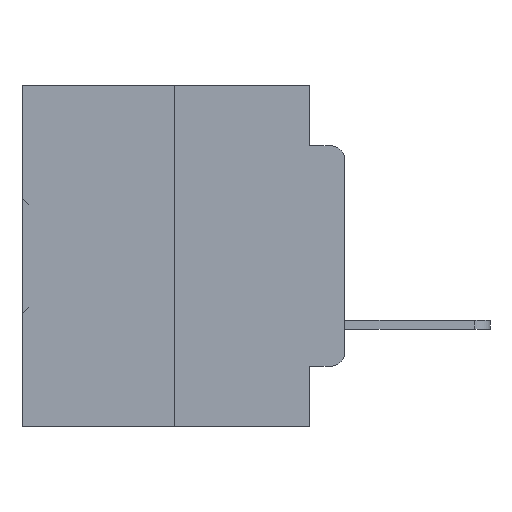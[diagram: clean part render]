
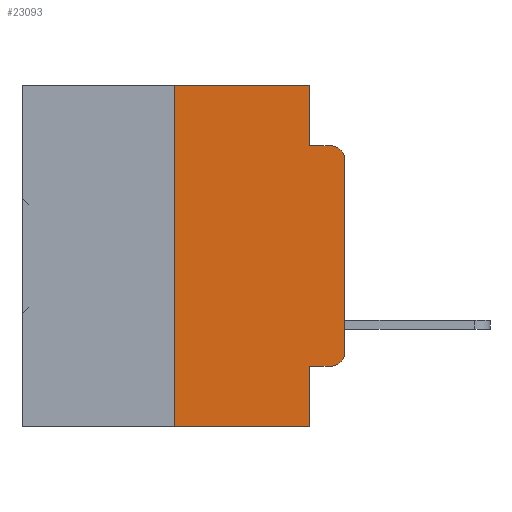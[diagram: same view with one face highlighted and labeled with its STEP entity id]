
A CAD part, left-side view. The second image highlights one B-rep face of the part: STEP entity #23093.
In plain terms, the highlighted planar face has unit normal (-1, 0, 0).
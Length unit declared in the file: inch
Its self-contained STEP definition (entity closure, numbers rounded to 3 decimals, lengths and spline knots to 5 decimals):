
#101 = ORIENTED_EDGE ( 'NONE', *, *, #20485, .T. ) ;
#163 = EDGE_CURVE ( 'NONE', #13387, #16653, #19277, .T. ) ;
#534 = ORIENTED_EDGE ( 'NONE', *, *, #12224, .T. ) ;
#1407 = ORIENTED_EDGE ( 'NONE', *, *, #3550, .F. ) ;
#1460 = LINE ( 'NONE', #19119, #8581 ) ;
#1593 = CARTESIAN_POINT ( 'NONE',  ( 0., 0.051, -0.5 ) ) ;
#1614 = ORIENTED_EDGE ( 'NONE', *, *, #21613, .F. ) ;
#1692 = ORIENTED_EDGE ( 'NONE', *, *, #24259, .F. ) ;
#1952 = ORIENTED_EDGE ( 'NONE', *, *, #17841, .F. ) ;
#2042 = ORIENTED_EDGE ( 'NONE', *, *, #13165, .T. ) ;
#2542 = DIRECTION ( 'NONE',  ( 0., 0., -1. ) ) ;
#2817 = ORIENTED_EDGE ( 'NONE', *, *, #163, .F. ) ;
#2893 = ORIENTED_EDGE ( 'NONE', *, *, #14076, .T. ) ;
#3377 = ORIENTED_EDGE ( 'NONE', *, *, #25380, .T. ) ;
#3550 = EDGE_CURVE ( 'NONE', #28048, #8764, #31536, .T. ) ;
#4096 = CARTESIAN_POINT ( 'NONE',  ( 0., 0.051, -0.0885 ) ) ;
#4329 = VECTOR ( 'NONE', #29502, 39.37008 ) ;
#5026 = CARTESIAN_POINT ( 'NONE',  ( 0., 0.02, -0.4115 ) ) ;
#5465 = CARTESIAN_POINT ( 'NONE',  ( 0., 0.051, -0.0885 ) ) ;
#6001 = VECTOR ( 'NONE', #16373, 39.37008 ) ;
#6758 = CARTESIAN_POINT ( 'NONE',  ( 0., 0.25, -0.5 ) ) ;
#6966 = CARTESIAN_POINT ( 'NONE',  ( 0., 0.051, 0. ) ) ;
#7599 = FACE_OUTER_BOUND ( 'NONE', #13425, .T. ) ;
#8366 = CARTESIAN_POINT ( 'NONE',  ( 0., 0.051, 0. ) ) ;
#8581 = VECTOR ( 'NONE', #27427, 39.37008 ) ;
#8764 = VERTEX_POINT ( 'NONE', #12356 ) ;
#8953 = VECTOR ( 'NONE', #23841, 39.37008 ) ;
#9687 = CARTESIAN_POINT ( 'NONE',  ( 0., 0., -0.3915 ) ) ;
#9900 = LINE ( 'NONE', #29376, #8953 ) ;
#11595 = CARTESIAN_POINT ( 'NONE',  ( 0., 0.02, -0.3915 ) ) ;
#11869 = VERTEX_POINT ( 'NONE', #6758 ) ;
#12214 = CARTESIAN_POINT ( 'NONE',  ( 0., 0.473, 0. ) ) ;
#12224 = EDGE_CURVE ( 'NONE', #22399, #8764, #19757, .T. ) ;
#12356 = CARTESIAN_POINT ( 'NONE',  ( 0., 0.02, -0.0885 ) ) ;
#12906 = CARTESIAN_POINT ( 'NONE',  ( 0., 0.473, 0. ) ) ;
#13165 = EDGE_CURVE ( 'NONE', #11869, #16653, #34197, .T. ) ;
#13387 = VERTEX_POINT ( 'NONE', #35613 ) ;
#13425 = EDGE_LOOP ( 'NONE', ( #101, #534, #1407, #1614, #1692, #1952, #2042, #2817, #2893, #3377 ) ) ;
#13742 = LINE ( 'NONE', #32911, #6001 ) ;
#14076 = EDGE_CURVE ( 'NONE', #13387, #35954, #20490, .T. ) ;
#14393 = DIRECTION ( 'NONE',  ( 0., 0., -1. ) ) ;
#14446 = CARTESIAN_POINT ( 'NONE',  ( 0., 0.051, -0.4115 ) ) ;
#15016 = DIRECTION ( 'NONE',  ( 0., -1., 0. ) ) ;
#15813 = DIRECTION ( 'NONE',  ( 0., 0., -1. ) ) ;
#16373 = DIRECTION ( 'NONE',  ( 0., 0., 1. ) ) ;
#16653 = VERTEX_POINT ( 'NONE', #1593 ) ;
#17252 = DIRECTION ( 'NONE',  ( 0., -1., 0. ) ) ;
#17841 = EDGE_CURVE ( 'NONE', #11869, #24341, #13742, .T. ) ;
#19119 = CARTESIAN_POINT ( 'NONE',  ( 0., 0., 0. ) ) ;
#19135 = VERTEX_POINT ( 'NONE', #6966 ) ;
#19277 = LINE ( 'NONE', #8366, #25858 ) ;
#19757 = CIRCLE ( 'NONE', #25357, 0.02 ) ;
#19957 = DIRECTION ( 'NONE',  ( -1., 0., 0. ) ) ;
#20037 = VECTOR ( 'NONE', #15016, 39.37008 ) ;
#20485 = EDGE_CURVE ( 'NONE', #29592, #22399, #1460, .T. ) ;
#20490 = LINE ( 'NONE', #14446, #34130 ) ;
#21199 = DIRECTION ( 'NONE',  ( 0., 0., -1. ) ) ;
#21613 = EDGE_CURVE ( 'NONE', #19135, #28048, #9900, .T. ) ;
#22399 = VERTEX_POINT ( 'NONE', #29401 ) ;
#23093 = ADVANCED_FACE ( 'NONE', ( #7599 ), #29711, .F. ) ;
#23841 = DIRECTION ( 'NONE',  ( 0., 0., -1. ) ) ;
#23976 = CARTESIAN_POINT ( 'NONE',  ( 0., 0.473, -0.5 ) ) ;
#24179 = DIRECTION ( 'NONE',  ( 0., -1., 0. ) ) ;
#24259 = EDGE_CURVE ( 'NONE', #24341, #19135, #34546, .T. ) ;
#24288 = VECTOR ( 'NONE', #24179, 39.37008 ) ;
#24341 = VERTEX_POINT ( 'NONE', #29156 ) ;
#25357 = AXIS2_PLACEMENT_3D ( 'NONE', #36249, #19957, #2542 ) ;
#25380 = EDGE_CURVE ( 'NONE', #35954, #29592, #36547, .T. ) ;
#25858 = VECTOR ( 'NONE', #21199, 39.37008 ) ;
#26328 = AXIS2_PLACEMENT_3D ( 'NONE', #11595, #31036, #14393 ) ;
#27427 = DIRECTION ( 'NONE',  ( 0., 0., 1. ) ) ;
#28048 = VERTEX_POINT ( 'NONE', #5465 ) ;
#29156 = CARTESIAN_POINT ( 'NONE',  ( 0., 0.25, 0. ) ) ;
#29376 = CARTESIAN_POINT ( 'NONE',  ( 0., 0.051, 0. ) ) ;
#29401 = CARTESIAN_POINT ( 'NONE',  ( 0., 0., -0.1085 ) ) ;
#29502 = DIRECTION ( 'NONE',  ( 0., -1., 0. ) ) ;
#29592 = VERTEX_POINT ( 'NONE', #9687 ) ;
#29711 = PLANE ( 'NONE',  #32165 ) ;
#31036 = DIRECTION ( 'NONE',  ( -1., 0., 0. ) ) ;
#31536 = LINE ( 'NONE', #4096, #24288 ) ;
#32165 = AXIS2_PLACEMENT_3D ( 'NONE', #12906, #32388, #15813 ) ;
#32388 = DIRECTION ( 'NONE',  ( 1., 0., 0. ) ) ;
#32911 = CARTESIAN_POINT ( 'NONE',  ( 0., 0.25, 0. ) ) ;
#34130 = VECTOR ( 'NONE', #17252, 39.37008 ) ;
#34197 = LINE ( 'NONE', #23976, #4329 ) ;
#34546 = LINE ( 'NONE', #12214, #20037 ) ;
#35613 = CARTESIAN_POINT ( 'NONE',  ( 0., 0.051, -0.4115 ) ) ;
#35954 = VERTEX_POINT ( 'NONE', #5026 ) ;
#36249 = CARTESIAN_POINT ( 'NONE',  ( 0., 0.02, -0.1085 ) ) ;
#36547 = CIRCLE ( 'NONE', #26328, 0.02 ) ;
